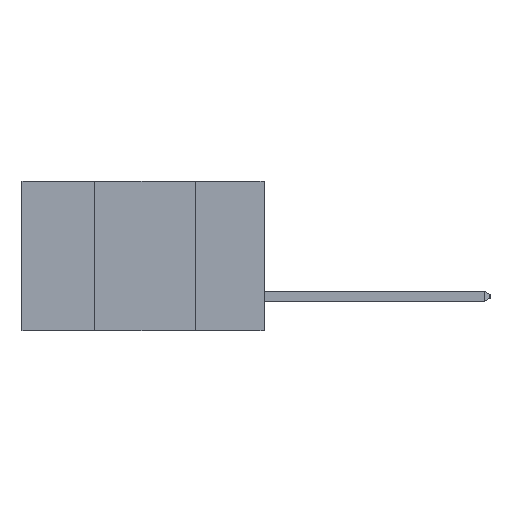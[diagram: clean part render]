
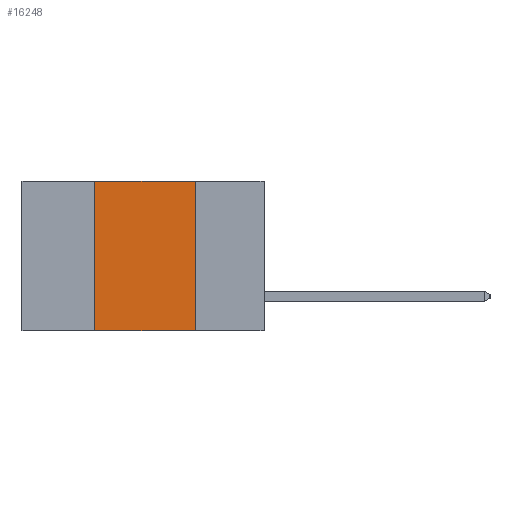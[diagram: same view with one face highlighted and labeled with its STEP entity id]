
A CAD part, left-side view. The second image highlights one B-rep face of the part: STEP entity #16248.
In plain terms, the highlighted planar face has unit normal (-1, 0, 0).
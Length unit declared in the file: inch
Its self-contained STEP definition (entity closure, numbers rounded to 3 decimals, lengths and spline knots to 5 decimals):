
#303 = VECTOR ( 'NONE', #737, 39.37008 ) ;
#367 = CARTESIAN_POINT ( 'NONE',  ( 0., 0.6, 0. ) ) ;
#737 = DIRECTION ( 'NONE',  ( 0., 0., -1. ) ) ;
#1489 = CARTESIAN_POINT ( 'NONE',  ( 0., 0.42, -0.37 ) ) ;
#1533 = VERTEX_POINT ( 'NONE', #8945 ) ;
#2042 = CARTESIAN_POINT ( 'NONE',  ( 0., 0.6, -0.37 ) ) ;
#2483 = VECTOR ( 'NONE', #13746, 39.37008 ) ;
#2617 = FACE_OUTER_BOUND ( 'NONE', #13776, .T. ) ;
#3247 = VERTEX_POINT ( 'NONE', #14745 ) ;
#3322 = LINE ( 'NONE', #9498, #303 ) ;
#4729 = ORIENTED_EDGE ( 'NONE', *, *, #11829, .F. ) ;
#4772 = VECTOR ( 'NONE', #10959, 39.37008 ) ;
#6223 = PLANE ( 'NONE',  #13219 ) ;
#7113 = CARTESIAN_POINT ( 'NONE',  ( 0., 0.17, -0.37 ) ) ;
#7683 = DIRECTION ( 'NONE',  ( 1., 0., 0. ) ) ;
#8017 = CARTESIAN_POINT ( 'NONE',  ( 0., 0.42, 0. ) ) ;
#8124 = ORIENTED_EDGE ( 'NONE', *, *, #15351, .F. ) ;
#8945 = CARTESIAN_POINT ( 'NONE',  ( 0., 0.17, 0. ) ) ;
#9498 = CARTESIAN_POINT ( 'NONE',  ( 0., 0.17, 0. ) ) ;
#9867 = EDGE_CURVE ( 'NONE', #14459, #11490, #17147, .T. ) ;
#10959 = DIRECTION ( 'NONE',  ( 0., 0., 1. ) ) ;
#11490 = VERTEX_POINT ( 'NONE', #7113 ) ;
#11829 = EDGE_CURVE ( 'NONE', #14459, #3247, #13032, .T. ) ;
#13032 = LINE ( 'NONE', #8017, #4772 ) ;
#13219 = AXIS2_PLACEMENT_3D ( 'NONE', #367, #7683, #18012 ) ;
#13746 = DIRECTION ( 'NONE',  ( 0., -1., 0. ) ) ;
#13776 = EDGE_LOOP ( 'NONE', ( #16002, #8124, #4729, #18743 ) ) ;
#14459 = VERTEX_POINT ( 'NONE', #1489 ) ;
#14745 = CARTESIAN_POINT ( 'NONE',  ( 0., 0.42, 0. ) ) ;
#15042 = VECTOR ( 'NONE', #18515, 39.37008 ) ;
#15351 = EDGE_CURVE ( 'NONE', #3247, #1533, #18927, .T. ) ;
#15595 = CARTESIAN_POINT ( 'NONE',  ( 0., 0.6, 0. ) ) ;
#15817 = EDGE_CURVE ( 'NONE', #1533, #11490, #3322, .T. ) ;
#16002 = ORIENTED_EDGE ( 'NONE', *, *, #15817, .F. ) ;
#16248 = ADVANCED_FACE ( 'NONE', ( #2617 ), #6223, .F. ) ;
#17147 = LINE ( 'NONE', #2042, #2483 ) ;
#18012 = DIRECTION ( 'NONE',  ( 0., 0., -1. ) ) ;
#18515 = DIRECTION ( 'NONE',  ( 0., -1., 0. ) ) ;
#18743 = ORIENTED_EDGE ( 'NONE', *, *, #9867, .T. ) ;
#18927 = LINE ( 'NONE', #15595, #15042 ) ;
